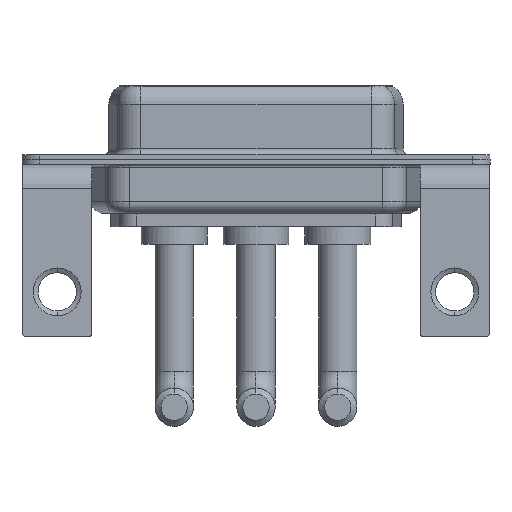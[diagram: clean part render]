
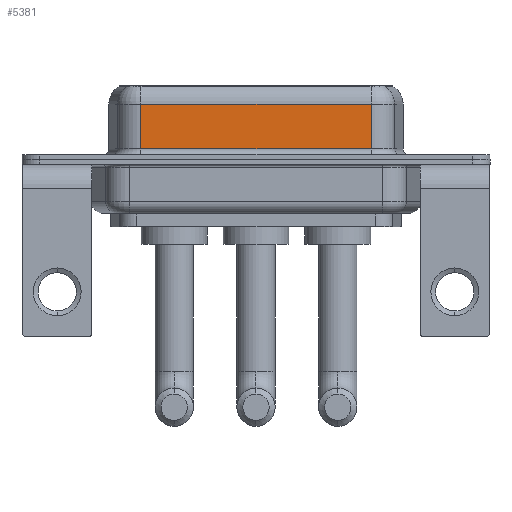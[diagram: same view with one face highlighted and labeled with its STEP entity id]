
A CAD part, front view. The second image highlights one B-rep face of the part: STEP entity #5381.
In plain terms, the highlighted planar face has unit normal (0, -1, 0).
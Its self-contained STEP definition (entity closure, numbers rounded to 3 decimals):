
#187 = VECTOR ( 'NONE', #5623, 1000. ) ;
#267 = DIRECTION ( 'NONE',  ( 0., 1., 0. ) ) ;
#545 = VERTEX_POINT ( 'NONE', #12027 ) ;
#617 = CARTESIAN_POINT ( 'NONE',  ( 26.287, -3.95, 4.65 ) ) ;
#620 = VECTOR ( 'NONE', #11432, 1000. ) ;
#981 = EDGE_LOOP ( 'NONE', ( #11640, #3782, #5100, #9187 ) ) ;
#1823 = EDGE_CURVE ( 'NONE', #7436, #11059, #7688, .T. ) ;
#2847 = CARTESIAN_POINT ( 'NONE',  ( 26.287, -3.95, 0.9 ) ) ;
#3085 = VECTOR ( 'NONE', #6753, 1000. ) ;
#3185 = CARTESIAN_POINT ( 'NONE',  ( 7.013, -3.95, 4.65 ) ) ;
#3628 = EDGE_CURVE ( 'NONE', #545, #10638, #7613, .T. ) ;
#3782 = ORIENTED_EDGE ( 'NONE', *, *, #1823, .T. ) ;
#4148 = CARTESIAN_POINT ( 'NONE',  ( 26.287, -3.95, 4.65 ) ) ;
#5100 = ORIENTED_EDGE ( 'NONE', *, *, #11981, .T. ) ;
#5336 = CARTESIAN_POINT ( 'NONE',  ( 26.287, -3.95, 6.4 ) ) ;
#5381 = ADVANCED_FACE ( 'NONE', ( #8400 ), #7395, .F. ) ;
#5623 = DIRECTION ( 'NONE',  ( 1., 0., 0. ) ) ;
#6223 = CARTESIAN_POINT ( 'NONE',  ( 26.287, -3.95, 0.9 ) ) ;
#6397 = CARTESIAN_POINT ( 'NONE',  ( 26.287, -3.95, 6.4 ) ) ;
#6753 = DIRECTION ( 'NONE',  ( -1., 0., 0. ) ) ;
#7395 = PLANE ( 'NONE',  #9523 ) ;
#7436 = VERTEX_POINT ( 'NONE', #4148 ) ;
#7486 = LINE ( 'NONE', #11565, #620 ) ;
#7613 = LINE ( 'NONE', #2847, #187 ) ;
#7688 = LINE ( 'NONE', #617, #3085 ) ;
#8400 = FACE_OUTER_BOUND ( 'NONE', #981, .T. ) ;
#9187 = ORIENTED_EDGE ( 'NONE', *, *, #3628, .T. ) ;
#9382 = DIRECTION ( 'NONE',  ( 0., 0., -1. ) ) ;
#9523 = AXIS2_PLACEMENT_3D ( 'NONE', #6397, #267, #10461 ) ;
#10384 = LINE ( 'NONE', #5336, #10982 ) ;
#10461 = DIRECTION ( 'NONE',  ( 0., 0., 1. ) ) ;
#10638 = VERTEX_POINT ( 'NONE', #6223 ) ;
#10982 = VECTOR ( 'NONE', #9382, 1000. ) ;
#11059 = VERTEX_POINT ( 'NONE', #3185 ) ;
#11432 = DIRECTION ( 'NONE',  ( 0., 0., -1. ) ) ;
#11565 = CARTESIAN_POINT ( 'NONE',  ( 7.013, -3.95, 6.4 ) ) ;
#11610 = EDGE_CURVE ( 'NONE', #7436, #10638, #10384, .T. ) ;
#11640 = ORIENTED_EDGE ( 'NONE', *, *, #11610, .F. ) ;
#11981 = EDGE_CURVE ( 'NONE', #11059, #545, #7486, .T. ) ;
#12027 = CARTESIAN_POINT ( 'NONE',  ( 7.013, -3.95, 0.9 ) ) ;
